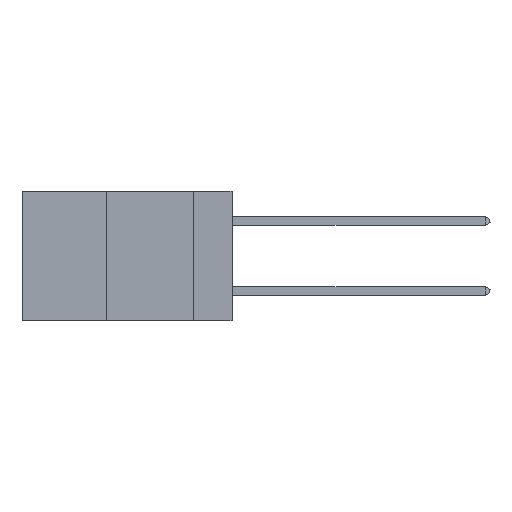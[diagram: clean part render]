
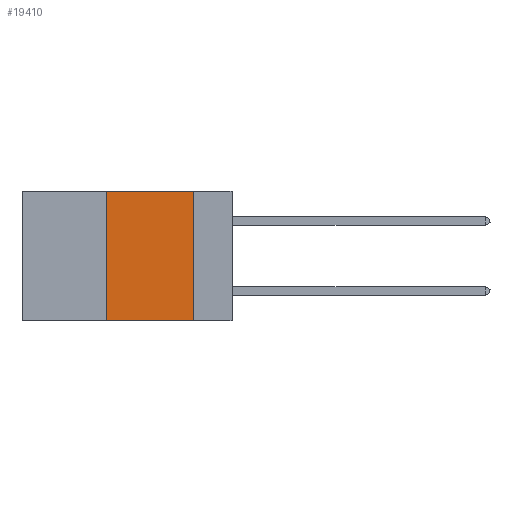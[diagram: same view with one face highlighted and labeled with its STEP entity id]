
A CAD part, left-side view. The second image highlights one B-rep face of the part: STEP entity #19410.
In plain terms, the highlighted planar face has unit normal (-1, 0, 0).
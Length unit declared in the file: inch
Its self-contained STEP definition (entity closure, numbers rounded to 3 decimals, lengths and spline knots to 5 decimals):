
#551 = EDGE_CURVE ( 'NONE', #15117, #24966, #34182, .T. ) ;
#782 = EDGE_CURVE ( 'NONE', #2999, #21056, #9889, .T. ) ;
#2999 = VERTEX_POINT ( 'NONE', #33954 ) ;
#3419 = LINE ( 'NONE', #19836, #18040 ) ;
#3918 = CARTESIAN_POINT ( 'NONE',  ( 0., 0.6, -0.37 ) ) ;
#6069 = DIRECTION ( 'NONE',  ( 1., 0., 0. ) ) ;
#6177 = AXIS2_PLACEMENT_3D ( 'NONE', #20496, #6069, #26255 ) ;
#6746 = EDGE_CURVE ( 'NONE', #21056, #24966, #31080, .T. ) ;
#9889 = LINE ( 'NONE', #24100, #31943 ) ;
#11315 = FACE_OUTER_BOUND ( 'NONE', #35780, .T. ) ;
#13383 = DIRECTION ( 'NONE',  ( 0., 0., -1. ) ) ;
#15117 = VERTEX_POINT ( 'NONE', #25324 ) ;
#16246 = ORIENTED_EDGE ( 'NONE', *, *, #27459, .F. ) ;
#18037 = VECTOR ( 'NONE', #26585, 39.37008 ) ;
#18040 = VECTOR ( 'NONE', #22694, 39.37008 ) ;
#18045 = ORIENTED_EDGE ( 'NONE', *, *, #551, .T. ) ;
#19410 = ADVANCED_FACE ( 'NONE', ( #11315 ), #31933, .F. ) ;
#19836 = CARTESIAN_POINT ( 'NONE',  ( 0., 0.36, 0. ) ) ;
#20496 = CARTESIAN_POINT ( 'NONE',  ( 0., 0.6, 0. ) ) ;
#21056 = VERTEX_POINT ( 'NONE', #30801 ) ;
#22694 = DIRECTION ( 'NONE',  ( 0., 0., 1. ) ) ;
#24100 = CARTESIAN_POINT ( 'NONE',  ( 0., 0.6, 0. ) ) ;
#24292 = ORIENTED_EDGE ( 'NONE', *, *, #782, .F. ) ;
#24966 = VERTEX_POINT ( 'NONE', #28655 ) ;
#25324 = CARTESIAN_POINT ( 'NONE',  ( 0., 0.36, -0.37 ) ) ;
#26255 = DIRECTION ( 'NONE',  ( 0., 0., -1. ) ) ;
#26585 = DIRECTION ( 'NONE',  ( 0., -1., 0. ) ) ;
#27459 = EDGE_CURVE ( 'NONE', #15117, #2999, #3419, .T. ) ;
#27854 = DIRECTION ( 'NONE',  ( 0., -1., 0. ) ) ;
#28655 = CARTESIAN_POINT ( 'NONE',  ( 0., 0.11, -0.37 ) ) ;
#30190 = VECTOR ( 'NONE', #13383, 39.37008 ) ;
#30609 = CARTESIAN_POINT ( 'NONE',  ( 0., 0.11, 0. ) ) ;
#30801 = CARTESIAN_POINT ( 'NONE',  ( 0., 0.11, 0. ) ) ;
#31080 = LINE ( 'NONE', #30609, #30190 ) ;
#31933 = PLANE ( 'NONE',  #6177 ) ;
#31943 = VECTOR ( 'NONE', #27854, 39.37008 ) ;
#33954 = CARTESIAN_POINT ( 'NONE',  ( 0., 0.36, 0. ) ) ;
#34182 = LINE ( 'NONE', #3918, #18037 ) ;
#34594 = ORIENTED_EDGE ( 'NONE', *, *, #6746, .F. ) ;
#35780 = EDGE_LOOP ( 'NONE', ( #34594, #24292, #16246, #18045 ) ) ;
